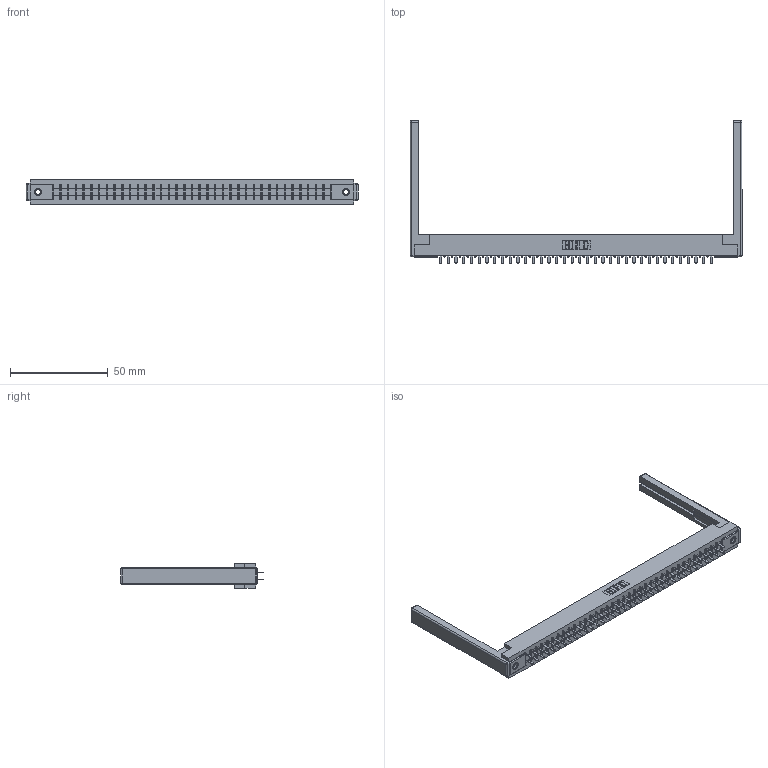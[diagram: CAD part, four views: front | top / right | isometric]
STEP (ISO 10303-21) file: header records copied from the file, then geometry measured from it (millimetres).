
FILE_DESCRIPTION (( 'STEP AP203' ), '1' );
FILE_NAME ('305-072-521-568.STEP', '2019-09-10T06:16:25', ( '' ), ( '' ), 'SwSTEP 2.0', 'SolidWorks 2016', '' );
FILE_SCHEMA (( 'CONFIG_CONTROL_DESIGN' ));
Length unit declared in the file: inch
Products named in the file (5): 307-220-068; 305 Part_.156 Dia; 305-290-001_521; 305-072-521-568; 345-250-001_345-250-001-102
Assembly tree (77 placements, depth 2):
  305-072-521-568
    305 Part_.156 Dia
    305-290-001_521  x72
    345-250-001_345-250-001-102  x2
    307-220-068  x2
Bounding box: 170.08 x 73.15 x 12.7 mm (x, y, z)
Volume: 21532 mm3; surface area: 26098.2 mm2
Topology: 77 solids, 77 shells, 3582 faces, 10174 edges, 6568 vertices
Faces by surface type: plane 2100, cylinder 1314, sphere 152, cone 12, torus 4
Entity records: 42348 total; most frequent: CARTESIAN_POINT 6979, ORIENTED_EDGE 6918, DIRECTION 6775, EDGE_CURVE 3459, VECTOR 2783, LINE 2783, VERTEX_POINT 2200, AXIS2_PLACEMENT_3D 1996
